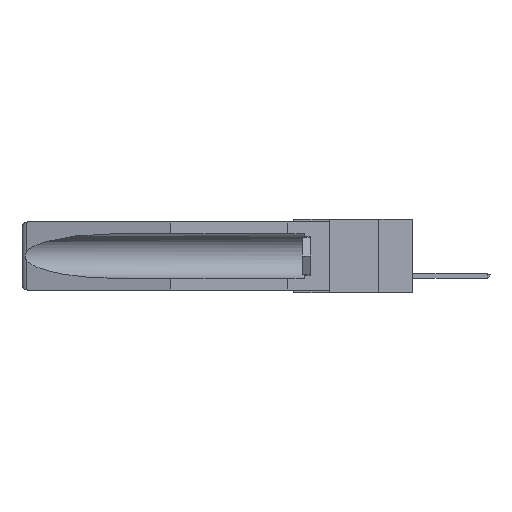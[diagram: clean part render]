
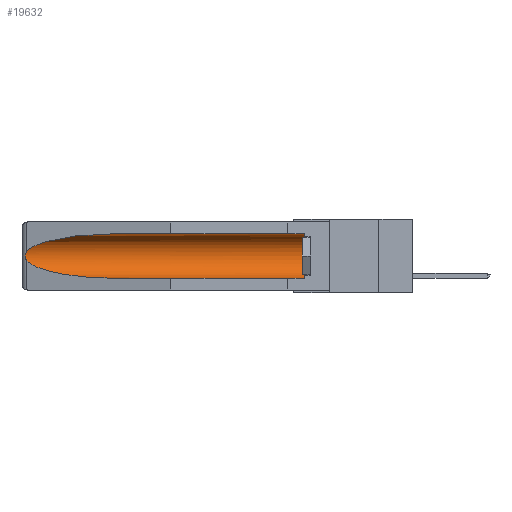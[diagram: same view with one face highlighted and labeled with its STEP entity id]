
A CAD part, left-side view. The second image highlights one B-rep face of the part: STEP entity #19632.
In plain terms, the highlighted cylindrical face has radius 2.857 mm (diameter 5.715 mm), a partial arc.
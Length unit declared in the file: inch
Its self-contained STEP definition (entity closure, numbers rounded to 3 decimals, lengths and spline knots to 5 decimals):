
#68 = EDGE_LOOP ( 'NONE', ( #30367, #20998, #9530, #5181, #14138, #12820 ) ) ;
#128 = CARTESIAN_POINT ( 'NONE',  ( 0.155, -0.30754, -0.059 ) ) ;
#240 = AXIS2_PLACEMENT_3D ( 'NONE', #11580, #25784, #4310 ) ;
#1207 = CARTESIAN_POINT ( 'NONE',  ( 0.155, 1.07973, -0.059 ) ) ;
#2200 = CARTESIAN_POINT ( 'NONE',  ( 0.2675, 1.53308, -0.16763 ) ) ;
#2308 = CARTESIAN_POINT ( 'NONE',  ( 0.26537, 1.52718, -0.14972 ) ) ;
#2321 = VERTEX_POINT ( 'NONE', #26373 ) ;
#2692 = CARTESIAN_POINT ( 'NONE',  ( 0.155, 1.07973, -0.284 ) ) ;
#2827 = CARTESIAN_POINT ( 'NONE',  ( 0.155, -0.30754, -0.284 ) ) ;
#3240 = CARTESIAN_POINT ( 'NONE',  ( 0.155, 0.126, -0.059 ) ) ;
#4310 = DIRECTION ( 'NONE',  ( 0., 0., 1. ) ) ;
#4481 = CARTESIAN_POINT ( 'NONE',  ( 0.26537, 1.52718, -0.14972 ) ) ;
#4656 = CARTESIAN_POINT ( 'NONE',  ( 0.2673, 1.53269, -0.17917 ) ) ;
#4743 = VERTEX_POINT ( 'NONE', #3240 ) ;
#5181 = ORIENTED_EDGE ( 'NONE', *, *, #28261, .F. ) ;
#5250 = DIRECTION ( 'NONE',  ( 0., 1., 0. ) ) ;
#5256 = CIRCLE ( 'NONE', #240, 0.1125 ) ;
#6464 = LINE ( 'NONE', #2827, #21937 ) ;
#6471 = EDGE_CURVE ( 'NONE', #4743, #14607, #25848, .T. ) ;
#7207 = CARTESIAN_POINT ( 'NONE',  ( 0.2675, 1.53308, -0.17534 ) ) ;
#8491 = VECTOR ( 'NONE', #5250, 39.37008 ) ;
#8648 = EDGE_CURVE ( 'NONE', #17923, #2321, #8997, .T. ) ;
#8997 =( BOUNDED_CURVE ( )  B_SPLINE_CURVE ( 3, ( #14733, #27038, #19712, #2692 ),
 .UNSPECIFIED., .F., .F. ) 
 B_SPLINE_CURVE_WITH_KNOTS ( ( 4, 4 ),
 ( 0.1948, 1.5708 ),
 .UNSPECIFIED. ) 
 CURVE ( )  GEOMETRIC_REPRESENTATION_ITEM ( )  RATIONAL_B_SPLINE_CURVE ( ( 1., 0.848, 0.848, 1. ) ) 
 REPRESENTATION_ITEM ( '' )  );
#9520 = CARTESIAN_POINT ( 'NONE',  ( 0.26597, 1.52961, -0.15275 ) ) ;
#9530 = ORIENTED_EDGE ( 'NONE', *, *, #8648, .T. ) ;
#10556 = EDGE_CURVE ( 'NONE', #16777, #17923, #14188, .T. ) ;
#11580 = CARTESIAN_POINT ( 'NONE',  ( 0.155, 0.126, -0.1715 ) ) ;
#11652 = CARTESIAN_POINT ( 'NONE',  ( 0.21114, 1.30732, -0.059 ) ) ;
#11923 = CARTESIAN_POINT ( 'NONE',  ( 0.2673, 1.5327, -0.16383 ) ) ;
#12199 = CYLINDRICAL_SURFACE ( 'NONE', #22418, 0.1125 ) ;
#12820 = ORIENTED_EDGE ( 'NONE', *, *, #6471, .T. ) ;
#14138 = ORIENTED_EDGE ( 'NONE', *, *, #31322, .T. ) ;
#14188 = B_SPLINE_CURVE_WITH_KNOTS ( 'NONE', 3,
 ( #2308, #9520, #16679, #11923, #2200, #7207, #4656, #19116, #21546, #16897 ),
 .UNSPECIFIED., .F., .F.,
 ( 4, 2, 2, 2, 4 ),
 ( 0., 0.00029, 0.00058, 0.00087, 0.00117 ),
 .UNSPECIFIED. ) ;
#14607 = VERTEX_POINT ( 'NONE', #1207 ) ;
#14733 = CARTESIAN_POINT ( 'NONE',  ( 0.26537, 1.52718, -0.19328 ) ) ;
#16410 = CARTESIAN_POINT ( 'NONE',  ( 0.155, 1.07973, -0.059 ) ) ;
#16511 = EDGE_CURVE ( 'NONE', #14607, #16777, #23883, .T. ) ;
#16679 = CARTESIAN_POINT ( 'NONE',  ( 0.26654, 1.53092, -0.15636 ) ) ;
#16777 = VERTEX_POINT ( 'NONE', #22663 ) ;
#16897 = CARTESIAN_POINT ( 'NONE',  ( 0.26537, 1.52718, -0.19328 ) ) ;
#17923 = VERTEX_POINT ( 'NONE', #23267 ) ;
#19116 = CARTESIAN_POINT ( 'NONE',  ( 0.26655, 1.53094, -0.18657 ) ) ;
#19156 = CARTESIAN_POINT ( 'NONE',  ( 0.25451, 1.48313, -0.09465 ) ) ;
#19445 = CARTESIAN_POINT ( 'NONE',  ( 0.155, 0.126, -0.284 ) ) ;
#19632 = ADVANCED_FACE ( 'NONE', ( #22787 ), #12199, .F. ) ;
#19712 = CARTESIAN_POINT ( 'NONE',  ( 0.21114, 1.30732, -0.284 ) ) ;
#20998 = ORIENTED_EDGE ( 'NONE', *, *, #10556, .T. ) ;
#21166 = DIRECTION ( 'NONE',  ( 0., 1., 0. ) ) ;
#21546 = CARTESIAN_POINT ( 'NONE',  ( 0.26597, 1.5296, -0.19026 ) ) ;
#21937 = VECTOR ( 'NONE', #29141, 39.37008 ) ;
#22418 = AXIS2_PLACEMENT_3D ( 'NONE', #25948, #21166, #23068 ) ;
#22663 = CARTESIAN_POINT ( 'NONE',  ( 0.26537, 1.52718, -0.14972 ) ) ;
#22787 = FACE_OUTER_BOUND ( 'NONE', #68, .T. ) ;
#23068 = DIRECTION ( 'NONE',  ( 0., 0., 1. ) ) ;
#23267 = CARTESIAN_POINT ( 'NONE',  ( 0.26537, 1.52718, -0.19328 ) ) ;
#23883 =( BOUNDED_CURVE ( )  B_SPLINE_CURVE ( 3, ( #16410, #11652, #19156, #4481 ),
 .UNSPECIFIED., .F., .F. ) 
 B_SPLINE_CURVE_WITH_KNOTS ( ( 4, 4 ),
 ( 4.71239, 6.08839 ),
 .UNSPECIFIED. ) 
 CURVE ( )  GEOMETRIC_REPRESENTATION_ITEM ( )  RATIONAL_B_SPLINE_CURVE ( ( 1., 0.848, 0.848, 1. ) ) 
 REPRESENTATION_ITEM ( '' )  );
#25784 = DIRECTION ( 'NONE',  ( 0., -1., 0. ) ) ;
#25848 = LINE ( 'NONE', #128, #8491 ) ;
#25948 = CARTESIAN_POINT ( 'NONE',  ( 0.155, -0.30754, -0.1715 ) ) ;
#26373 = CARTESIAN_POINT ( 'NONE',  ( 0.155, 1.07973, -0.284 ) ) ;
#26751 = VERTEX_POINT ( 'NONE', #19445 ) ;
#27038 = CARTESIAN_POINT ( 'NONE',  ( 0.25451, 1.48313, -0.24835 ) ) ;
#28261 = EDGE_CURVE ( 'NONE', #26751, #2321, #6464, .T. ) ;
#29141 = DIRECTION ( 'NONE',  ( 0., 1., 0. ) ) ;
#30367 = ORIENTED_EDGE ( 'NONE', *, *, #16511, .T. ) ;
#31322 = EDGE_CURVE ( 'NONE', #26751, #4743, #5256, .T. ) ;
